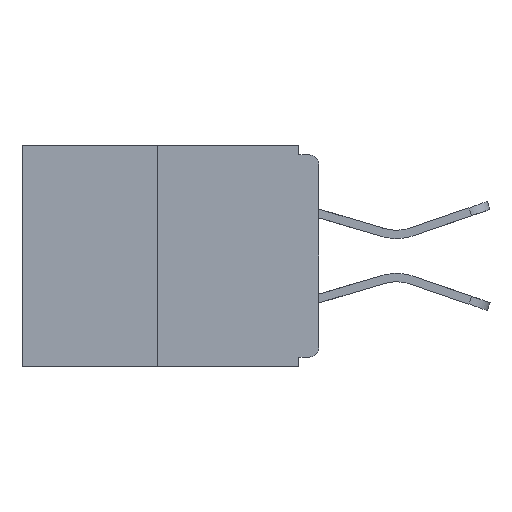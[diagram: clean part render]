
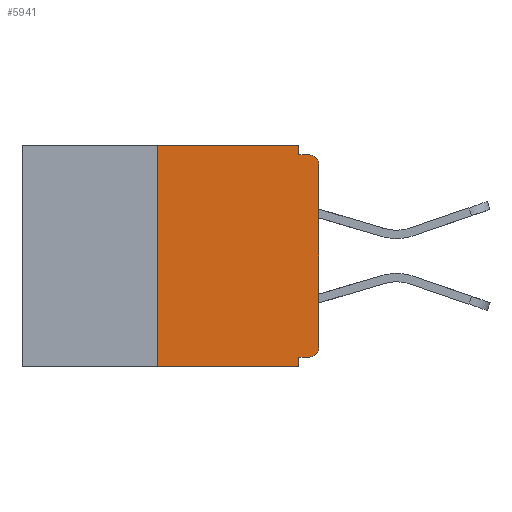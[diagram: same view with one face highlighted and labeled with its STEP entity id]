
A CAD part, left-side view. The second image highlights one B-rep face of the part: STEP entity #5941.
In plain terms, the highlighted planar face has unit normal (-1, 0, 0).
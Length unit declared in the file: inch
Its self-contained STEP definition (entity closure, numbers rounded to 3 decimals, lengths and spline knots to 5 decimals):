
#197 = ORIENTED_EDGE ( 'NONE', *, *, #17680, .F. ) ;
#299 = EDGE_CURVE ( 'NONE', #7914, #12593, #11577, .T. ) ;
#534 = ORIENTED_EDGE ( 'NONE', *, *, #15672, .F. ) ;
#1498 = EDGE_CURVE ( 'NONE', #12620, #16465, #18202, .T. ) ;
#1707 = VERTEX_POINT ( 'NONE', #6711 ) ;
#1929 = ORIENTED_EDGE ( 'NONE', *, *, #7101, .F. ) ;
#2220 = DIRECTION ( 'NONE',  ( 0., -1., 0. ) ) ;
#2301 = EDGE_LOOP ( 'NONE', ( #17537, #534, #11831, #5758, #1929, #2797, #17289, #16658, #197, #17332 ) ) ;
#2797 = ORIENTED_EDGE ( 'NONE', *, *, #5749, .T. ) ;
#3575 = CARTESIAN_POINT ( 'NONE',  ( 0., 0.46, -0.343 ) ) ;
#3671 = VECTOR ( 'NONE', #17037, 39.37008 ) ;
#3677 = VECTOR ( 'NONE', #12649, 39.37008 ) ;
#4532 = LINE ( 'NONE', #12712, #3677 ) ;
#4609 = DIRECTION ( 'NONE',  ( -1., 0., 0. ) ) ;
#4646 = AXIS2_PLACEMENT_3D ( 'NONE', #15915, #14110, #7002 ) ;
#5342 = EDGE_CURVE ( 'NONE', #13371, #13403, #10731, .T. ) ;
#5749 = EDGE_CURVE ( 'NONE', #12038, #7993, #17375, .T. ) ;
#5758 = ORIENTED_EDGE ( 'NONE', *, *, #299, .F. ) ;
#5778 = CARTESIAN_POINT ( 'NONE',  ( 0., 0., -0.03 ) ) ;
#5805 = CARTESIAN_POINT ( 'NONE',  ( 0., 0.031, -0.015 ) ) ;
#5829 = FACE_OUTER_BOUND ( 'NONE', #2301, .T. ) ;
#5941 = ADVANCED_FACE ( 'NONE', ( #5829 ), #16538, .F. ) ;
#6053 = CARTESIAN_POINT ( 'NONE',  ( 0., 0.25, 0. ) ) ;
#6096 = DIRECTION ( 'NONE',  ( 0., 1., 0. ) ) ;
#6402 = CARTESIAN_POINT ( 'NONE',  ( 0., 0.015, -0.015 ) ) ;
#6455 = DIRECTION ( 'NONE',  ( 1., 0., 0. ) ) ;
#6505 = DIRECTION ( 'NONE',  ( 0., -1., 0. ) ) ;
#6517 = DIRECTION ( 'NONE',  ( 0., 0., -1. ) ) ;
#6711 = CARTESIAN_POINT ( 'NONE',  ( 0., 0.25, -0.343 ) ) ;
#6996 = EDGE_CURVE ( 'NONE', #7993, #12620, #8257, .T. ) ;
#7002 = DIRECTION ( 'NONE',  ( 0., 0., -1. ) ) ;
#7077 = CARTESIAN_POINT ( 'NONE',  ( 0., 0.031, -0.343 ) ) ;
#7101 = EDGE_CURVE ( 'NONE', #12038, #7914, #12873, .T. ) ;
#7118 = CARTESIAN_POINT ( 'NONE',  ( 0., 0.031, -0.343 ) ) ;
#7385 = VECTOR ( 'NONE', #6505, 39.37008 ) ;
#7525 = CARTESIAN_POINT ( 'NONE',  ( 0., 0.031, 0. ) ) ;
#7891 = VERTEX_POINT ( 'NONE', #5805 ) ;
#7914 = VERTEX_POINT ( 'NONE', #13400 ) ;
#7993 = VERTEX_POINT ( 'NONE', #12233 ) ;
#8257 = LINE ( 'NONE', #18047, #15118 ) ;
#8323 = AXIS2_PLACEMENT_3D ( 'NONE', #17846, #6455, #6517 ) ;
#8908 = CARTESIAN_POINT ( 'NONE',  ( 0., 0.015, -0.03 ) ) ;
#9133 = VECTOR ( 'NONE', #6096, 39.37008 ) ;
#9237 = DIRECTION ( 'NONE',  ( 0., 0., -1. ) ) ;
#10003 = LINE ( 'NONE', #3575, #7385 ) ;
#10731 = LINE ( 'NONE', #17439, #15145 ) ;
#11577 = LINE ( 'NONE', #7118, #3671 ) ;
#11831 = ORIENTED_EDGE ( 'NONE', *, *, #17609, .T. ) ;
#11904 = VECTOR ( 'NONE', #9237, 39.37008 ) ;
#12038 = VERTEX_POINT ( 'NONE', #16032 ) ;
#12233 = CARTESIAN_POINT ( 'NONE',  ( 0., 0., -0.313 ) ) ;
#12593 = VERTEX_POINT ( 'NONE', #7077 ) ;
#12620 = VERTEX_POINT ( 'NONE', #5778 ) ;
#12649 = DIRECTION ( 'NONE',  ( 0., -1., 0. ) ) ;
#12712 = CARTESIAN_POINT ( 'NONE',  ( 0., 0., -0.015 ) ) ;
#12873 = LINE ( 'NONE', #13107, #9133 ) ;
#13107 = CARTESIAN_POINT ( 'NONE',  ( 0., 0., -0.328 ) ) ;
#13217 = LINE ( 'NONE', #13631, #11904 ) ;
#13371 = VERTEX_POINT ( 'NONE', #6053 ) ;
#13400 = CARTESIAN_POINT ( 'NONE',  ( 0., 0.031, -0.328 ) ) ;
#13403 = VERTEX_POINT ( 'NONE', #7525 ) ;
#13631 = CARTESIAN_POINT ( 'NONE',  ( 0., 0.031, 0. ) ) ;
#14110 = DIRECTION ( 'NONE',  ( -1., 0., 0. ) ) ;
#14282 = AXIS2_PLACEMENT_3D ( 'NONE', #8908, #4609, #16037 ) ;
#14737 = DIRECTION ( 'NONE',  ( 0., 0., 1. ) ) ;
#14751 = EDGE_CURVE ( 'NONE', #13403, #7891, #13217, .T. ) ;
#15118 = VECTOR ( 'NONE', #16847, 39.37008 ) ;
#15145 = VECTOR ( 'NONE', #2220, 39.37008 ) ;
#15195 = VECTOR ( 'NONE', #14737, 39.37008 ) ;
#15672 = EDGE_CURVE ( 'NONE', #1707, #13371, #15853, .T. ) ;
#15853 = LINE ( 'NONE', #17673, #15195 ) ;
#15915 = CARTESIAN_POINT ( 'NONE',  ( 0., 0.015, -0.313 ) ) ;
#16032 = CARTESIAN_POINT ( 'NONE',  ( 0., 0.015, -0.328 ) ) ;
#16037 = DIRECTION ( 'NONE',  ( 0., 0., -1. ) ) ;
#16465 = VERTEX_POINT ( 'NONE', #6402 ) ;
#16538 = PLANE ( 'NONE',  #8323 ) ;
#16658 = ORIENTED_EDGE ( 'NONE', *, *, #1498, .T. ) ;
#16847 = DIRECTION ( 'NONE',  ( 0., 0., 1. ) ) ;
#17037 = DIRECTION ( 'NONE',  ( 0., 0., -1. ) ) ;
#17289 = ORIENTED_EDGE ( 'NONE', *, *, #6996, .T. ) ;
#17332 = ORIENTED_EDGE ( 'NONE', *, *, #14751, .F. ) ;
#17375 = CIRCLE ( 'NONE', #4646, 0.015 ) ;
#17439 = CARTESIAN_POINT ( 'NONE',  ( 0., 0.46, 0. ) ) ;
#17537 = ORIENTED_EDGE ( 'NONE', *, *, #5342, .F. ) ;
#17609 = EDGE_CURVE ( 'NONE', #1707, #12593, #10003, .T. ) ;
#17673 = CARTESIAN_POINT ( 'NONE',  ( 0., 0.25, 0. ) ) ;
#17680 = EDGE_CURVE ( 'NONE', #7891, #16465, #4532, .T. ) ;
#17846 = CARTESIAN_POINT ( 'NONE',  ( 0., 0.46, 0. ) ) ;
#18047 = CARTESIAN_POINT ( 'NONE',  ( 0., 0., 0. ) ) ;
#18202 = CIRCLE ( 'NONE', #14282, 0.015 ) ;
